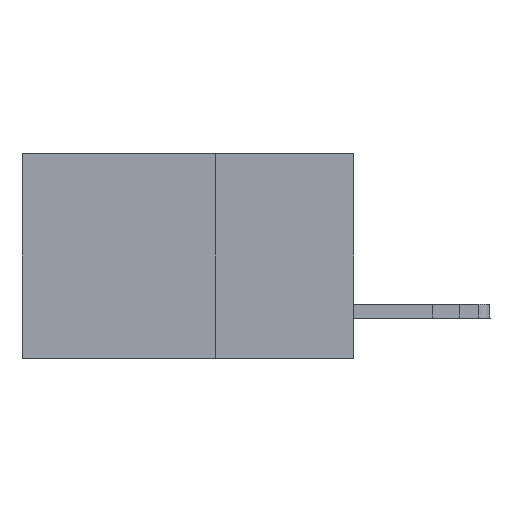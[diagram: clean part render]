
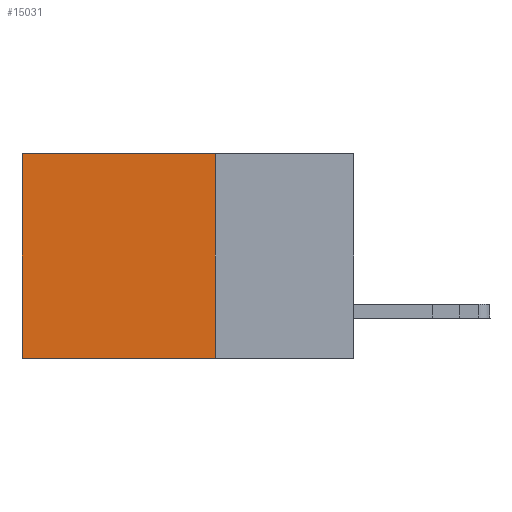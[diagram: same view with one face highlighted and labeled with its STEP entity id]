
A CAD part, left-side view. The second image highlights one B-rep face of the part: STEP entity #15031.
In plain terms, the highlighted planar face has unit normal (-1, 0, 0).
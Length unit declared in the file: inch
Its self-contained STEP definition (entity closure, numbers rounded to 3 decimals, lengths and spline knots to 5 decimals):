
#360 = CARTESIAN_POINT ( 'NONE',  ( 0.2875, 0.25, 0. ) ) ;
#1943 = VECTOR ( 'NONE', #22865, 39.37008 ) ;
#2175 = VECTOR ( 'NONE', #7233, 39.37008 ) ;
#2232 = CARTESIAN_POINT ( 'NONE',  ( 0.2875, 0.6, 0. ) ) ;
#2462 = ORIENTED_EDGE ( 'NONE', *, *, #15611, .T. ) ;
#3081 = DIRECTION ( 'NONE',  ( 0., 1., 0. ) ) ;
#5196 = DIRECTION ( 'NONE',  ( 0., 0., -1. ) ) ;
#7233 = DIRECTION ( 'NONE',  ( 0., 1., 0. ) ) ;
#7427 = PLANE ( 'NONE',  #12902 ) ;
#8165 = ORIENTED_EDGE ( 'NONE', *, *, #14331, .F. ) ;
#8352 = CARTESIAN_POINT ( 'NONE',  ( 0.2875, 0.25, -0.37 ) ) ;
#9343 = DIRECTION ( 'NONE',  ( 1., 0., 0. ) ) ;
#11218 = LINE ( 'NONE', #14703, #16354 ) ;
#11368 = ORIENTED_EDGE ( 'NONE', *, *, #24261, .F. ) ;
#11461 = ORIENTED_EDGE ( 'NONE', *, *, #14514, .T. ) ;
#12902 = AXIS2_PLACEMENT_3D ( 'NONE', #20788, #9343, #22693 ) ;
#13323 = LINE ( 'NONE', #16682, #23458 ) ;
#14331 = EDGE_CURVE ( 'NONE', #19020, #23587, #11218, .T. ) ;
#14514 = EDGE_CURVE ( 'NONE', #17071, #23587, #18428, .T. ) ;
#14703 = CARTESIAN_POINT ( 'NONE',  ( 0.2875, 0.25, -0.37 ) ) ;
#14820 = CARTESIAN_POINT ( 'NONE',  ( 0.2875, 0.25, 0. ) ) ;
#15031 = ADVANCED_FACE ( 'NONE', ( #16009 ), #7427, .F. ) ;
#15611 = EDGE_CURVE ( 'NONE', #20894, #17071, #18068, .T. ) ;
#16009 = FACE_OUTER_BOUND ( 'NONE', #16417, .T. ) ;
#16354 = VECTOR ( 'NONE', #3081, 39.37008 ) ;
#16417 = EDGE_LOOP ( 'NONE', ( #11461, #8165, #11368, #2462 ) ) ;
#16682 = CARTESIAN_POINT ( 'NONE',  ( 0.2875, 0.25, 0. ) ) ;
#17071 = VERTEX_POINT ( 'NONE', #2232 ) ;
#18068 = LINE ( 'NONE', #14820, #2175 ) ;
#18428 = LINE ( 'NONE', #20972, #1943 ) ;
#19020 = VERTEX_POINT ( 'NONE', #8352 ) ;
#20788 = CARTESIAN_POINT ( 'NONE',  ( 0.2875, 0.25, 0. ) ) ;
#20894 = VERTEX_POINT ( 'NONE', #360 ) ;
#20972 = CARTESIAN_POINT ( 'NONE',  ( 0.2875, 0.6, 0. ) ) ;
#21912 = CARTESIAN_POINT ( 'NONE',  ( 0.2875, 0.6, -0.37 ) ) ;
#22693 = DIRECTION ( 'NONE',  ( 0., 0., -1. ) ) ;
#22865 = DIRECTION ( 'NONE',  ( 0., 0., -1. ) ) ;
#23458 = VECTOR ( 'NONE', #5196, 39.37008 ) ;
#23587 = VERTEX_POINT ( 'NONE', #21912 ) ;
#24261 = EDGE_CURVE ( 'NONE', #20894, #19020, #13323, .T. ) ;
